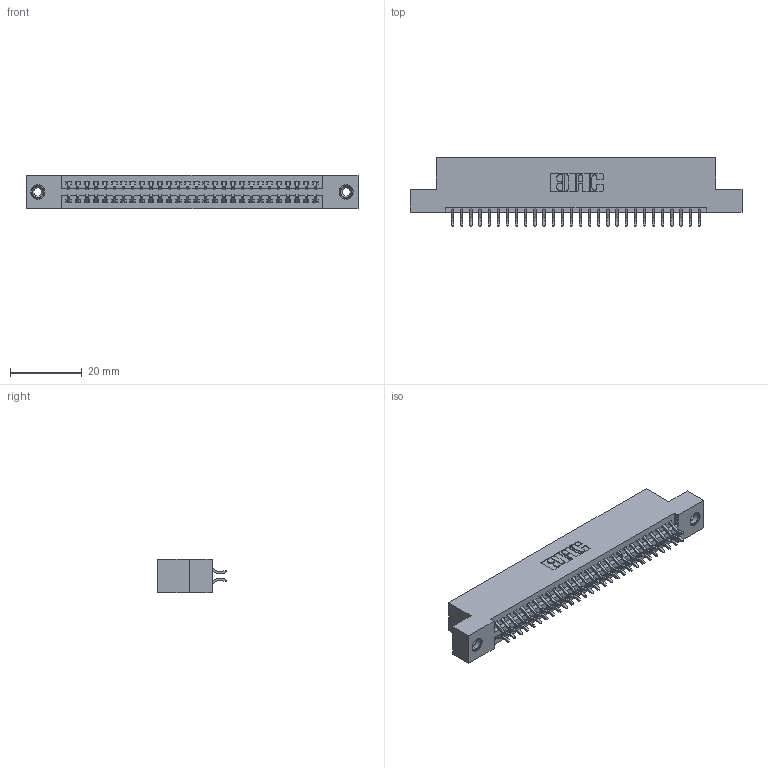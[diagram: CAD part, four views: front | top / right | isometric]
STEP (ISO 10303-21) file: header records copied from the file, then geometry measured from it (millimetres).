
FILE_DESCRIPTION (( 'STEP AP203' ), '1' );
FILE_NAME ('395-056-556-208.STEP', '2018-11-22T06:00:59', ( '' ), ( '' ), 'SwSTEP 2.0', 'SolidWorks 2016', '' );
FILE_SCHEMA (( 'CONFIG_CONTROL_DESIGN' ));
Length unit declared in the file: inch
Products named in the file (4): 345 Part_Flush Mounting Lugs - 0.156 Dia-TI; 345-292-001_556 Tail; 395-056-556-208; 345-250-001_345-250-003-102
Assembly tree (59 placements, depth 2):
  395-056-556-208
    345 Part_Flush Mounting Lugs - 0.156 Dia-TI
    345-292-001_556 Tail  x56
    345-250-001_345-250-003-102  x2
Bounding box: 92.33 x 19.24 x 9.4 mm (x, y, z)
Volume: 8830.2 mm3; surface area: 12745.8 mm2
Topology: 59 solids, 59 shells, 3322 faces, 9829 edges, 6470 vertices
Faces by surface type: plane 2184, cylinder 1122, cone 12, torus 4
Entity records: 25260 total; most frequent: CARTESIAN_POINT 4243, ORIENTED_EDGE 4158, DIRECTION 3773, EDGE_CURVE 2079, VECTOR 1807, LINE 1807, VERTEX_POINT 1380, AXIS2_PLACEMENT_3D 983
